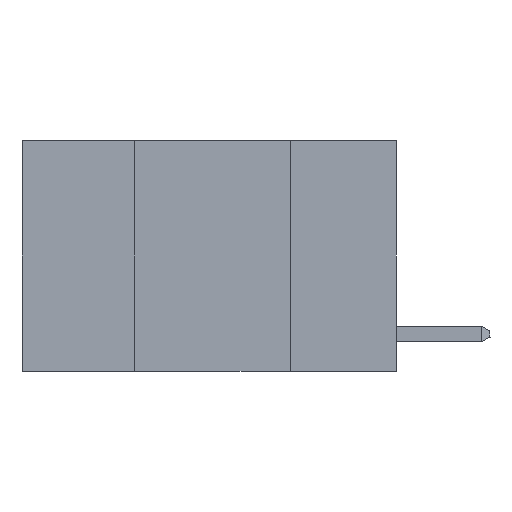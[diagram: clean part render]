
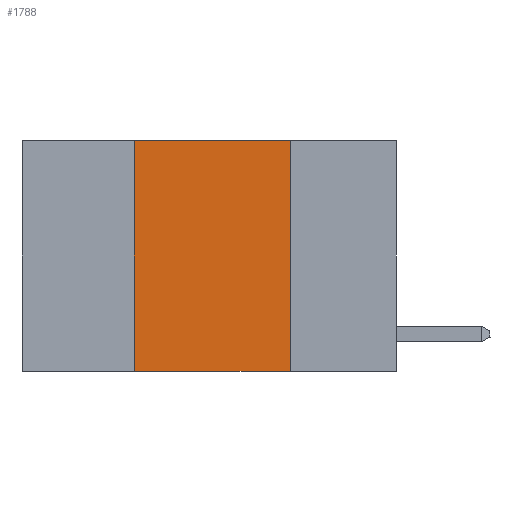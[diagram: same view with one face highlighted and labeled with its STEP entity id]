
A CAD part, left-side view. The second image highlights one B-rep face of the part: STEP entity #1788.
In plain terms, the highlighted planar face has unit normal (-1, 0, 0).
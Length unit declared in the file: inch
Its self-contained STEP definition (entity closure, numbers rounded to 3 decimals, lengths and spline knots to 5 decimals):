
#460 = LINE ( 'NONE', #8520, #13012 ) ;
#1076 = VECTOR ( 'NONE', #12226, 39.37008 ) ;
#1100 = CARTESIAN_POINT ( 'NONE',  ( 0., 0.42, 0. ) ) ;
#1324 = ORIENTED_EDGE ( 'NONE', *, *, #5848, .F. ) ;
#1453 = ORIENTED_EDGE ( 'NONE', *, *, #12192, .F. ) ;
#1713 = PLANE ( 'NONE',  #3472 ) ;
#1788 = ADVANCED_FACE ( 'NONE', ( #7800 ), #1713, .F. ) ;
#2270 = LINE ( 'NONE', #9382, #1076 ) ;
#2386 = DIRECTION ( 'NONE',  ( 0., 0., -1. ) ) ;
#2443 = LINE ( 'NONE', #3251, #12360 ) ;
#2712 = EDGE_CURVE ( 'NONE', #5056, #4014, #9984, .T. ) ;
#3251 = CARTESIAN_POINT ( 'NONE',  ( 0., 0.6, 0. ) ) ;
#3472 = AXIS2_PLACEMENT_3D ( 'NONE', #10789, #11724, #6918 ) ;
#3592 = VERTEX_POINT ( 'NONE', #4226 ) ;
#3787 = ORIENTED_EDGE ( 'NONE', *, *, #2712, .T. ) ;
#4014 = VERTEX_POINT ( 'NONE', #10973 ) ;
#4184 = ORIENTED_EDGE ( 'NONE', *, *, #10815, .F. ) ;
#4226 = CARTESIAN_POINT ( 'NONE',  ( 0., 0.17, 0. ) ) ;
#4930 = CARTESIAN_POINT ( 'NONE',  ( 0., 0.6, -0.37 ) ) ;
#5056 = VERTEX_POINT ( 'NONE', #11718 ) ;
#5403 = DIRECTION ( 'NONE',  ( 0., -1., 0. ) ) ;
#5582 = VECTOR ( 'NONE', #10766, 39.37008 ) ;
#5848 = EDGE_CURVE ( 'NONE', #5056, #11209, #2270, .T. ) ;
#6866 = EDGE_LOOP ( 'NONE', ( #1453, #4184, #1324, #3787 ) ) ;
#6918 = DIRECTION ( 'NONE',  ( 0., 0., -1. ) ) ;
#7800 = FACE_OUTER_BOUND ( 'NONE', #6866, .T. ) ;
#8520 = CARTESIAN_POINT ( 'NONE',  ( 0., 0.17, 0. ) ) ;
#9382 = CARTESIAN_POINT ( 'NONE',  ( 0., 0.42, 0. ) ) ;
#9984 = LINE ( 'NONE', #4930, #5582 ) ;
#10766 = DIRECTION ( 'NONE',  ( 0., -1., 0. ) ) ;
#10789 = CARTESIAN_POINT ( 'NONE',  ( 0., 0.6, 0. ) ) ;
#10815 = EDGE_CURVE ( 'NONE', #11209, #3592, #2443, .T. ) ;
#10973 = CARTESIAN_POINT ( 'NONE',  ( 0., 0.17, -0.37 ) ) ;
#11209 = VERTEX_POINT ( 'NONE', #1100 ) ;
#11718 = CARTESIAN_POINT ( 'NONE',  ( 0., 0.42, -0.37 ) ) ;
#11724 = DIRECTION ( 'NONE',  ( 1., 0., 0. ) ) ;
#12192 = EDGE_CURVE ( 'NONE', #3592, #4014, #460, .T. ) ;
#12226 = DIRECTION ( 'NONE',  ( 0., 0., 1. ) ) ;
#12360 = VECTOR ( 'NONE', #5403, 39.37008 ) ;
#13012 = VECTOR ( 'NONE', #2386, 39.37008 ) ;
